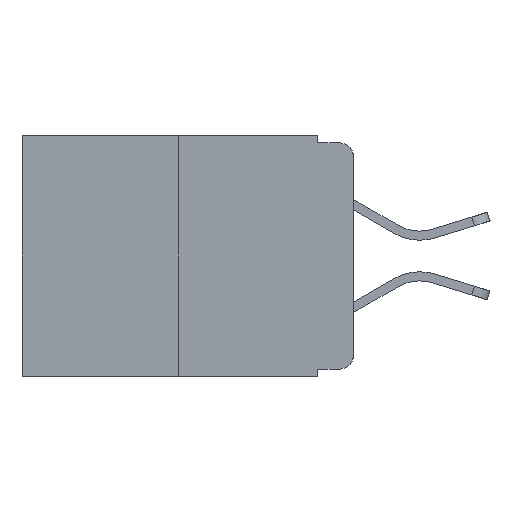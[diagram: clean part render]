
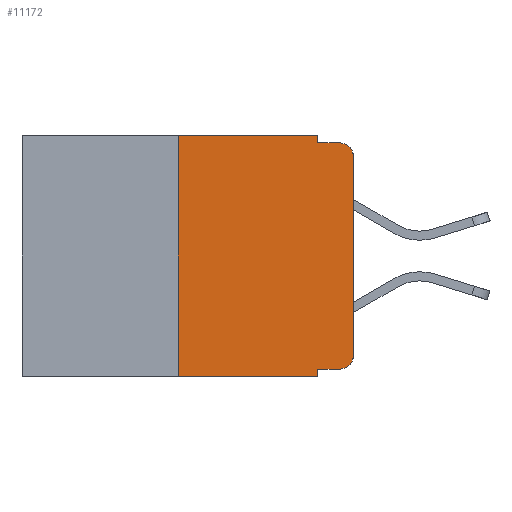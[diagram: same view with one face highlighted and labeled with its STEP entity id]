
A CAD part, left-side view. The second image highlights one B-rep face of the part: STEP entity #11172.
In plain terms, the highlighted planar face has unit normal (-1, 0, 0).
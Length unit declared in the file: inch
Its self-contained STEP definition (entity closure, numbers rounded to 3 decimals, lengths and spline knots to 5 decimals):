
#5 = EDGE_CURVE ( 'NONE', #788, #7102, #5616, .T. ) ;
#139 = DIRECTION ( 'NONE',  ( 0., 0., 1. ) ) ;
#388 = ORIENTED_EDGE ( 'NONE', *, *, #5, .T. ) ;
#788 = VERTEX_POINT ( 'NONE', #3683 ) ;
#973 = VERTEX_POINT ( 'NONE', #3426 ) ;
#1036 = VERTEX_POINT ( 'NONE', #5636 ) ;
#1084 = ORIENTED_EDGE ( 'NONE', *, *, #6494, .T. ) ;
#1190 = VERTEX_POINT ( 'NONE', #11818 ) ;
#1247 = ORIENTED_EDGE ( 'NONE', *, *, #7139, .F. ) ;
#1423 = LINE ( 'NONE', #5021, #6521 ) ;
#1822 = CARTESIAN_POINT ( 'NONE',  ( 0., 0.051, -0.01 ) ) ;
#2132 = EDGE_CURVE ( 'NONE', #10038, #788, #4960, .T. ) ;
#2192 = EDGE_LOOP ( 'NONE', ( #2549, #388, #5835, #4417, #2707, #6005, #3643, #1247, #1084, #7113 ) ) ;
#2529 = EDGE_CURVE ( 'NONE', #973, #11523, #6236, .T. ) ;
#2549 = ORIENTED_EDGE ( 'NONE', *, *, #2132, .T. ) ;
#2669 = DIRECTION ( 'NONE',  ( 0., -1., 0. ) ) ;
#2707 = ORIENTED_EDGE ( 'NONE', *, *, #2529, .F. ) ;
#2777 = CARTESIAN_POINT ( 'NONE',  ( 0., 0.473, 0. ) ) ;
#3122 = CARTESIAN_POINT ( 'NONE',  ( 0., 0.473, 0. ) ) ;
#3333 = CARTESIAN_POINT ( 'NONE',  ( 0., 0.051, -0.01 ) ) ;
#3336 = CARTESIAN_POINT ( 'NONE',  ( 0., 0., -0.313 ) ) ;
#3368 = DIRECTION ( 'NONE',  ( -1., 0., 0. ) ) ;
#3426 = CARTESIAN_POINT ( 'NONE',  ( 0., 0.25, 0. ) ) ;
#3643 = ORIENTED_EDGE ( 'NONE', *, *, #11927, .T. ) ;
#3667 = LINE ( 'NONE', #6433, #8731 ) ;
#3683 = CARTESIAN_POINT ( 'NONE',  ( 0., 0., -0.03 ) ) ;
#3908 = CARTESIAN_POINT ( 'NONE',  ( 0., 0.02, -0.01 ) ) ;
#4187 = AXIS2_PLACEMENT_3D ( 'NONE', #7519, #3368, #10660 ) ;
#4361 = VECTOR ( 'NONE', #12745, 39.37008 ) ;
#4417 = ORIENTED_EDGE ( 'NONE', *, *, #9847, .F. ) ;
#4630 = VECTOR ( 'NONE', #2669, 39.37008 ) ;
#4803 = CIRCLE ( 'NONE', #5232, 0.02 ) ;
#4906 = VERTEX_POINT ( 'NONE', #3333 ) ;
#4960 = LINE ( 'NONE', #12177, #10008 ) ;
#4969 = DIRECTION ( 'NONE',  ( 0., 0., -1. ) ) ;
#4989 = LINE ( 'NONE', #1822, #4361 ) ;
#5021 = CARTESIAN_POINT ( 'NONE',  ( 0., 0.051, 0. ) ) ;
#5232 = AXIS2_PLACEMENT_3D ( 'NONE', #6133, #12933, #7132 ) ;
#5376 = DIRECTION ( 'NONE',  ( 0., -1., 0. ) ) ;
#5616 = CIRCLE ( 'NONE', #4187, 0.02 ) ;
#5636 = CARTESIAN_POINT ( 'NONE',  ( 0., 0.051, -0.343 ) ) ;
#5791 = EDGE_CURVE ( 'NONE', #7420, #10038, #4803, .T. ) ;
#5835 = ORIENTED_EDGE ( 'NONE', *, *, #12390, .F. ) ;
#6005 = ORIENTED_EDGE ( 'NONE', *, *, #8509, .F. ) ;
#6054 = DIRECTION ( 'NONE',  ( 0., 0., -1. ) ) ;
#6133 = CARTESIAN_POINT ( 'NONE',  ( 0., 0.02, -0.313 ) ) ;
#6156 = DIRECTION ( 'NONE',  ( 1., 0., 0. ) ) ;
#6208 = VECTOR ( 'NONE', #4969, 39.37008 ) ;
#6236 = LINE ( 'NONE', #2777, #11202 ) ;
#6433 = CARTESIAN_POINT ( 'NONE',  ( 0., 0.25, 0. ) ) ;
#6494 = EDGE_CURVE ( 'NONE', #1190, #7420, #9993, .T. ) ;
#6521 = VECTOR ( 'NONE', #6054, 39.37008 ) ;
#7102 = VERTEX_POINT ( 'NONE', #3908 ) ;
#7113 = ORIENTED_EDGE ( 'NONE', *, *, #5791, .T. ) ;
#7132 = DIRECTION ( 'NONE',  ( 0., 0., -1. ) ) ;
#7139 = EDGE_CURVE ( 'NONE', #1190, #1036, #8890, .T. ) ;
#7365 = CARTESIAN_POINT ( 'NONE',  ( 0., 0.473, -0.343 ) ) ;
#7412 = DIRECTION ( 'NONE',  ( 0., 0., 1. ) ) ;
#7420 = VERTEX_POINT ( 'NONE', #12345 ) ;
#7519 = CARTESIAN_POINT ( 'NONE',  ( 0., 0.02, -0.03 ) ) ;
#7685 = LINE ( 'NONE', #7365, #12549 ) ;
#7908 = CARTESIAN_POINT ( 'NONE',  ( 0., 0.25, -0.343 ) ) ;
#8290 = AXIS2_PLACEMENT_3D ( 'NONE', #3122, #6156, #12954 ) ;
#8509 = EDGE_CURVE ( 'NONE', #9192, #973, #3667, .T. ) ;
#8707 = CARTESIAN_POINT ( 'NONE',  ( 0., 0.051, -0.333 ) ) ;
#8731 = VECTOR ( 'NONE', #7412, 39.37008 ) ;
#8890 = LINE ( 'NONE', #8991, #6208 ) ;
#8991 = CARTESIAN_POINT ( 'NONE',  ( 0., 0.051, 0. ) ) ;
#9128 = FACE_OUTER_BOUND ( 'NONE', #2192, .T. ) ;
#9192 = VERTEX_POINT ( 'NONE', #7908 ) ;
#9847 = EDGE_CURVE ( 'NONE', #11523, #4906, #1423, .T. ) ;
#9993 = LINE ( 'NONE', #8707, #4630 ) ;
#10008 = VECTOR ( 'NONE', #139, 39.37008 ) ;
#10038 = VERTEX_POINT ( 'NONE', #3336 ) ;
#10660 = DIRECTION ( 'NONE',  ( 0., 0., -1. ) ) ;
#11172 = ADVANCED_FACE ( 'NONE', ( #9128 ), #12000, .F. ) ;
#11202 = VECTOR ( 'NONE', #11720, 39.37008 ) ;
#11523 = VERTEX_POINT ( 'NONE', #11595 ) ;
#11595 = CARTESIAN_POINT ( 'NONE',  ( 0., 0.051, 0. ) ) ;
#11720 = DIRECTION ( 'NONE',  ( 0., -1., 0. ) ) ;
#11818 = CARTESIAN_POINT ( 'NONE',  ( 0., 0.051, -0.333 ) ) ;
#11927 = EDGE_CURVE ( 'NONE', #9192, #1036, #7685, .T. ) ;
#12000 = PLANE ( 'NONE',  #8290 ) ;
#12177 = CARTESIAN_POINT ( 'NONE',  ( 0., 0., 0. ) ) ;
#12345 = CARTESIAN_POINT ( 'NONE',  ( 0., 0.02, -0.333 ) ) ;
#12390 = EDGE_CURVE ( 'NONE', #4906, #7102, #4989, .T. ) ;
#12549 = VECTOR ( 'NONE', #5376, 39.37008 ) ;
#12745 = DIRECTION ( 'NONE',  ( 0., -1., 0. ) ) ;
#12933 = DIRECTION ( 'NONE',  ( -1., 0., 0. ) ) ;
#12954 = DIRECTION ( 'NONE',  ( 0., 0., -1. ) ) ;
